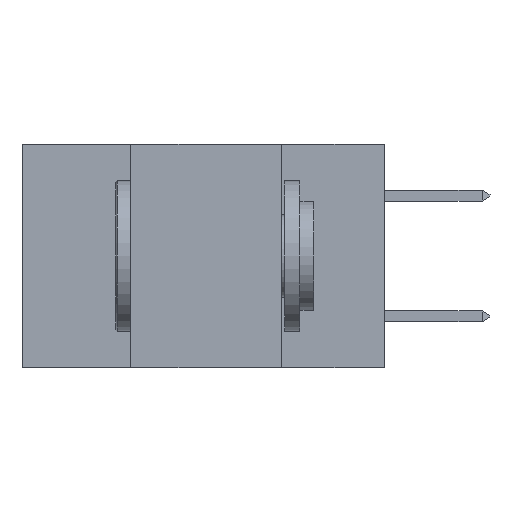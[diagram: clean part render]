
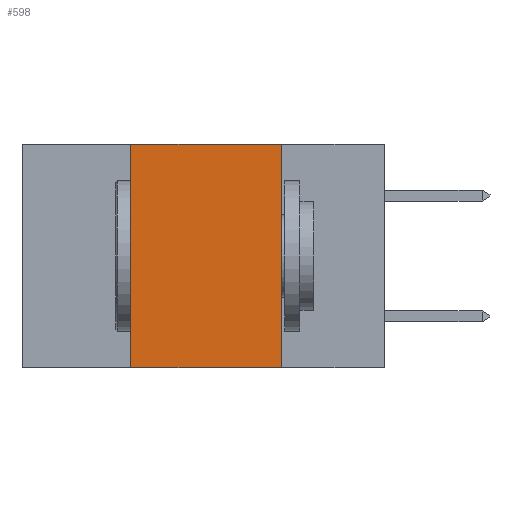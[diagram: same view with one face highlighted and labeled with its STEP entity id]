
A CAD part, left-side view. The second image highlights one B-rep face of the part: STEP entity #598.
In plain terms, the highlighted planar face has unit normal (-1, 0, 0).
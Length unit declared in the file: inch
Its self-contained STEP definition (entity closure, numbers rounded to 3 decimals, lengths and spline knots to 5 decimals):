
#598 = ADVANCED_FACE ( 'NONE', ( #17965 ), #2869, .F. ) ;
#935 = VECTOR ( 'NONE', #13880, 39.37008 ) ;
#1903 = CARTESIAN_POINT ( 'NONE',  ( 0., 0.17, -0.37 ) ) ;
#2030 = DIRECTION ( 'NONE',  ( 0., 0., 1. ) ) ;
#2164 = LINE ( 'NONE', #19790, #23046 ) ;
#2869 = PLANE ( 'NONE',  #24028 ) ;
#4177 = CARTESIAN_POINT ( 'NONE',  ( 0., 0.42, 0. ) ) ;
#4362 = LINE ( 'NONE', #23483, #20940 ) ;
#5369 = CARTESIAN_POINT ( 'NONE',  ( 0., 0.17, 0. ) ) ;
#5506 = ORIENTED_EDGE ( 'NONE', *, *, #17491, .T. ) ;
#5727 = ORIENTED_EDGE ( 'NONE', *, *, #18492, .F. ) ;
#5827 = CARTESIAN_POINT ( 'NONE',  ( 0., 0.42, -0.37 ) ) ;
#6770 = DIRECTION ( 'NONE',  ( 0., -1., 0. ) ) ;
#7094 = EDGE_CURVE ( 'NONE', #7484, #23747, #23055, .T. ) ;
#7484 = VERTEX_POINT ( 'NONE', #5369 ) ;
#10650 = DIRECTION ( 'NONE',  ( 0., 0., -1. ) ) ;
#10681 = CARTESIAN_POINT ( 'NONE',  ( 0., 0.6, -0.37 ) ) ;
#13880 = DIRECTION ( 'NONE',  ( 0., 0., -1. ) ) ;
#14714 = VECTOR ( 'NONE', #6770, 39.37008 ) ;
#14732 = CARTESIAN_POINT ( 'NONE',  ( 0., 0.6, 0. ) ) ;
#15083 = EDGE_CURVE ( 'NONE', #21467, #19613, #4362, .T. ) ;
#15938 = CARTESIAN_POINT ( 'NONE',  ( 0., 0.17, 0. ) ) ;
#17491 = EDGE_CURVE ( 'NONE', #21467, #23747, #23646, .T. ) ;
#17965 = FACE_OUTER_BOUND ( 'NONE', #18247, .T. ) ;
#18247 = EDGE_LOOP ( 'NONE', ( #22066, #5727, #20522, #5506 ) ) ;
#18492 = EDGE_CURVE ( 'NONE', #19613, #7484, #2164, .T. ) ;
#19613 = VERTEX_POINT ( 'NONE', #4177 ) ;
#19790 = CARTESIAN_POINT ( 'NONE',  ( 0., 0.6, 0. ) ) ;
#20522 = ORIENTED_EDGE ( 'NONE', *, *, #15083, .F. ) ;
#20940 = VECTOR ( 'NONE', #2030, 39.37008 ) ;
#21467 = VERTEX_POINT ( 'NONE', #5827 ) ;
#22066 = ORIENTED_EDGE ( 'NONE', *, *, #7094, .F. ) ;
#22188 = DIRECTION ( 'NONE',  ( 1., 0., 0. ) ) ;
#23046 = VECTOR ( 'NONE', #23992, 39.37008 ) ;
#23055 = LINE ( 'NONE', #15938, #935 ) ;
#23483 = CARTESIAN_POINT ( 'NONE',  ( 0., 0.42, 0. ) ) ;
#23646 = LINE ( 'NONE', #10681, #14714 ) ;
#23747 = VERTEX_POINT ( 'NONE', #1903 ) ;
#23992 = DIRECTION ( 'NONE',  ( 0., -1., 0. ) ) ;
#24028 = AXIS2_PLACEMENT_3D ( 'NONE', #14732, #22188, #10650 ) ;
